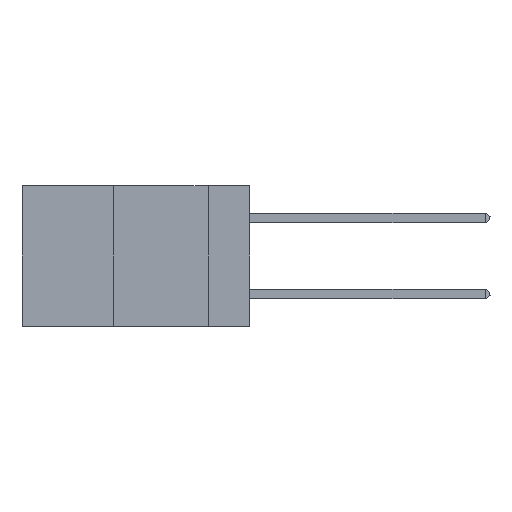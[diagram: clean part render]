
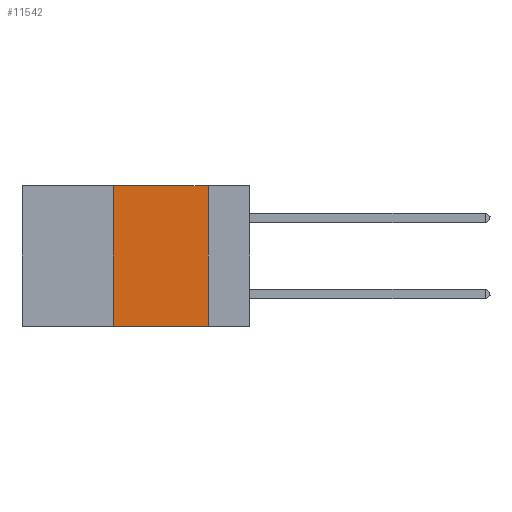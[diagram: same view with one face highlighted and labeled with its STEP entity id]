
A CAD part, left-side view. The second image highlights one B-rep face of the part: STEP entity #11542.
In plain terms, the highlighted planar face has unit normal (-1, 0, 0).
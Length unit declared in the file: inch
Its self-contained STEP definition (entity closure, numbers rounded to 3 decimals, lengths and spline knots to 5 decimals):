
#74 = CARTESIAN_POINT ( 'NONE',  ( 0., 0.6, 0. ) ) ;
#430 = CARTESIAN_POINT ( 'NONE',  ( 0., 0.11, 0. ) ) ;
#695 = AXIS2_PLACEMENT_3D ( 'NONE', #74, #14175, #4459 ) ;
#2736 = CARTESIAN_POINT ( 'NONE',  ( 0., 0.11, 0. ) ) ;
#3432 = EDGE_CURVE ( 'NONE', #23911, #3997, #14412, .T. ) ;
#3997 = VERTEX_POINT ( 'NONE', #13738 ) ;
#4001 = DIRECTION ( 'NONE',  ( 0., 0., 1. ) ) ;
#4459 = DIRECTION ( 'NONE',  ( 0., 0., -1. ) ) ;
#4660 = PLANE ( 'NONE',  #695 ) ;
#5468 = CARTESIAN_POINT ( 'NONE',  ( 0., 0.11, -0.37 ) ) ;
#5599 = CARTESIAN_POINT ( 'NONE',  ( 0., 0.6, 0. ) ) ;
#7187 = ORIENTED_EDGE ( 'NONE', *, *, #29188, .F. ) ;
#7377 = EDGE_LOOP ( 'NONE', ( #7788, #7187, #24790, #21128 ) ) ;
#7788 = ORIENTED_EDGE ( 'NONE', *, *, #25471, .F. ) ;
#8178 = VECTOR ( 'NONE', #4001, 39.37008 ) ;
#8821 = CARTESIAN_POINT ( 'NONE',  ( 0., 0.36, -0.37 ) ) ;
#11417 = FACE_OUTER_BOUND ( 'NONE', #7377, .T. ) ;
#11542 = ADVANCED_FACE ( 'NONE', ( #11417 ), #4660, .F. ) ;
#12860 = VERTEX_POINT ( 'NONE', #5468 ) ;
#13738 = CARTESIAN_POINT ( 'NONE',  ( 0., 0.36, 0. ) ) ;
#14175 = DIRECTION ( 'NONE',  ( 1., 0., 0. ) ) ;
#14412 = LINE ( 'NONE', #20717, #8178 ) ;
#15236 = VECTOR ( 'NONE', #15297, 39.37008 ) ;
#15297 = DIRECTION ( 'NONE',  ( 0., -1., 0. ) ) ;
#15880 = LINE ( 'NONE', #5599, #18115 ) ;
#16728 = LINE ( 'NONE', #27266, #15236 ) ;
#18048 = DIRECTION ( 'NONE',  ( 0., 0., -1. ) ) ;
#18115 = VECTOR ( 'NONE', #22119, 39.37008 ) ;
#19570 = LINE ( 'NONE', #430, #25103 ) ;
#20717 = CARTESIAN_POINT ( 'NONE',  ( 0., 0.36, 0. ) ) ;
#21128 = ORIENTED_EDGE ( 'NONE', *, *, #27933, .T. ) ;
#21132 = VERTEX_POINT ( 'NONE', #2736 ) ;
#22119 = DIRECTION ( 'NONE',  ( 0., -1., 0. ) ) ;
#23911 = VERTEX_POINT ( 'NONE', #8821 ) ;
#24790 = ORIENTED_EDGE ( 'NONE', *, *, #3432, .F. ) ;
#25103 = VECTOR ( 'NONE', #18048, 39.37008 ) ;
#25471 = EDGE_CURVE ( 'NONE', #21132, #12860, #19570, .T. ) ;
#27266 = CARTESIAN_POINT ( 'NONE',  ( 0., 0.6, -0.37 ) ) ;
#27933 = EDGE_CURVE ( 'NONE', #23911, #12860, #16728, .T. ) ;
#29188 = EDGE_CURVE ( 'NONE', #3997, #21132, #15880, .T. ) ;
